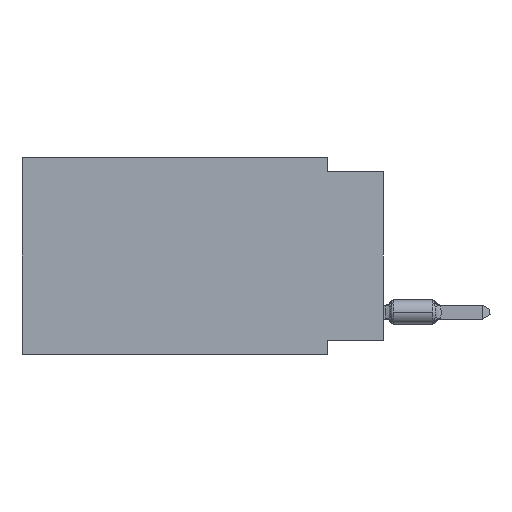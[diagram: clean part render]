
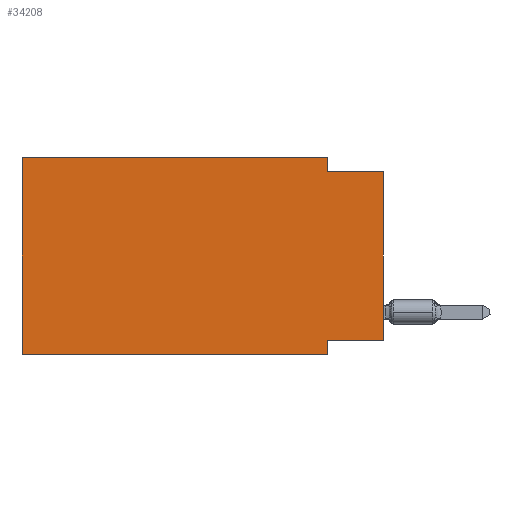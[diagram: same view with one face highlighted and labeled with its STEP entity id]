
A CAD part, left-side view. The second image highlights one B-rep face of the part: STEP entity #34208.
In plain terms, the highlighted planar face has unit normal (-1, 0, 0).
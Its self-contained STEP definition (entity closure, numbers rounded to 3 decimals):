
#397 = CARTESIAN_POINT ( 'NONE',  ( 0., 16.383, 0. ) ) ;
#1089 = CARTESIAN_POINT ( 'NONE',  ( 0., 2.54, -0.635 ) ) ;
#1188 = VERTEX_POINT ( 'NONE', #28321 ) ;
#2357 = VERTEX_POINT ( 'NONE', #41494 ) ;
#2854 = DIRECTION ( 'NONE',  ( 0., -1., 0. ) ) ;
#2933 = DIRECTION ( 'NONE',  ( 0., 0., 1. ) ) ;
#3095 = DIRECTION ( 'NONE',  ( 0., -1., 0. ) ) ;
#3100 = DIRECTION ( 'NONE',  ( 0., 0., -1. ) ) ;
#3881 = VERTEX_POINT ( 'NONE', #1089 ) ;
#4241 = LINE ( 'NONE', #31183, #39779 ) ;
#4692 = VECTOR ( 'NONE', #2854, 1000. ) ;
#6119 = LINE ( 'NONE', #16395, #36717 ) ;
#6169 = EDGE_LOOP ( 'NONE', ( #34546, #23011, #8400, #35651, #37942, #13078, #42358, #32319 ) ) ;
#6913 = VECTOR ( 'NONE', #18164, 1000. ) ;
#8400 = ORIENTED_EDGE ( 'NONE', *, *, #27381, .F. ) ;
#8729 = CARTESIAN_POINT ( 'NONE',  ( 0., 0., -8.255 ) ) ;
#10161 = DIRECTION ( 'NONE',  ( 0., 0., 1. ) ) ;
#10206 = CARTESIAN_POINT ( 'NONE',  ( 0., 16.383, -8.89 ) ) ;
#11511 = CARTESIAN_POINT ( 'NONE',  ( 0., 2.54, 0. ) ) ;
#12654 = DIRECTION ( 'NONE',  ( 1., 0., 0. ) ) ;
#13078 = ORIENTED_EDGE ( 'NONE', *, *, #33266, .T. ) ;
#13573 = LINE ( 'NONE', #27513, #36193 ) ;
#14473 = LINE ( 'NONE', #42339, #35614 ) ;
#15375 = EDGE_CURVE ( 'NONE', #3881, #1188, #6119, .T. ) ;
#15848 = CARTESIAN_POINT ( 'NONE',  ( 0., 16.383, 0. ) ) ;
#16395 = CARTESIAN_POINT ( 'NONE',  ( 0., 0., -0.635 ) ) ;
#16535 = VECTOR ( 'NONE', #2933, 1000. ) ;
#16970 = EDGE_CURVE ( 'NONE', #33494, #21144, #4241, .T. ) ;
#18164 = DIRECTION ( 'NONE',  ( 0., 0., -1. ) ) ;
#19035 = DIRECTION ( 'NONE',  ( 0., 0., -1. ) ) ;
#20432 = VERTEX_POINT ( 'NONE', #11511 ) ;
#21144 = VERTEX_POINT ( 'NONE', #28409 ) ;
#21553 = LINE ( 'NONE', #39148, #39898 ) ;
#22958 = CARTESIAN_POINT ( 'NONE',  ( 0., 2.54, -8.89 ) ) ;
#23011 = ORIENTED_EDGE ( 'NONE', *, *, #15375, .F. ) ;
#26921 = DIRECTION ( 'NONE',  ( 0., -1., 0. ) ) ;
#27381 = EDGE_CURVE ( 'NONE', #20432, #3881, #39830, .T. ) ;
#27513 = CARTESIAN_POINT ( 'NONE',  ( 0., 0., 0. ) ) ;
#28005 = AXIS2_PLACEMENT_3D ( 'NONE', #40522, #12654, #3100 ) ;
#28321 = CARTESIAN_POINT ( 'NONE',  ( 0., 0., -0.635 ) ) ;
#28409 = CARTESIAN_POINT ( 'NONE',  ( 0., 2.54, -8.255 ) ) ;
#28490 = VERTEX_POINT ( 'NONE', #10206 ) ;
#28647 = CARTESIAN_POINT ( 'NONE',  ( 0., 2.54, 0. ) ) ;
#29059 = VERTEX_POINT ( 'NONE', #22958 ) ;
#31183 = CARTESIAN_POINT ( 'NONE',  ( 0., 0., -8.255 ) ) ;
#32264 = EDGE_CURVE ( 'NONE', #21144, #29059, #21553, .T. ) ;
#32319 = ORIENTED_EDGE ( 'NONE', *, *, #16970, .F. ) ;
#33266 = EDGE_CURVE ( 'NONE', #28490, #29059, #14473, .T. ) ;
#33494 = VERTEX_POINT ( 'NONE', #8729 ) ;
#34208 = ADVANCED_FACE ( 'NONE', ( #36877 ), #37572, .F. ) ;
#34546 = ORIENTED_EDGE ( 'NONE', *, *, #42898, .T. ) ;
#34601 = DIRECTION ( 'NONE',  ( 0., 1., 0. ) ) ;
#34883 = LINE ( 'NONE', #397, #16535 ) ;
#34978 = EDGE_CURVE ( 'NONE', #2357, #20432, #40981, .T. ) ;
#35614 = VECTOR ( 'NONE', #3095, 1000. ) ;
#35651 = ORIENTED_EDGE ( 'NONE', *, *, #34978, .F. ) ;
#36193 = VECTOR ( 'NONE', #10161, 1000. ) ;
#36717 = VECTOR ( 'NONE', #26921, 1000. ) ;
#36877 = FACE_OUTER_BOUND ( 'NONE', #6169, .T. ) ;
#37572 = PLANE ( 'NONE',  #28005 ) ;
#37942 = ORIENTED_EDGE ( 'NONE', *, *, #43663, .F. ) ;
#39148 = CARTESIAN_POINT ( 'NONE',  ( 0., 2.54, -8.89 ) ) ;
#39779 = VECTOR ( 'NONE', #34601, 1000. ) ;
#39830 = LINE ( 'NONE', #28647, #6913 ) ;
#39898 = VECTOR ( 'NONE', #19035, 1000. ) ;
#40522 = CARTESIAN_POINT ( 'NONE',  ( 0., 16.383, 0. ) ) ;
#40981 = LINE ( 'NONE', #15848, #4692 ) ;
#41494 = CARTESIAN_POINT ( 'NONE',  ( 0., 16.383, 0. ) ) ;
#42339 = CARTESIAN_POINT ( 'NONE',  ( 0., 16.383, -8.89 ) ) ;
#42358 = ORIENTED_EDGE ( 'NONE', *, *, #32264, .F. ) ;
#42898 = EDGE_CURVE ( 'NONE', #33494, #1188, #13573, .T. ) ;
#43663 = EDGE_CURVE ( 'NONE', #28490, #2357, #34883, .T. ) ;
